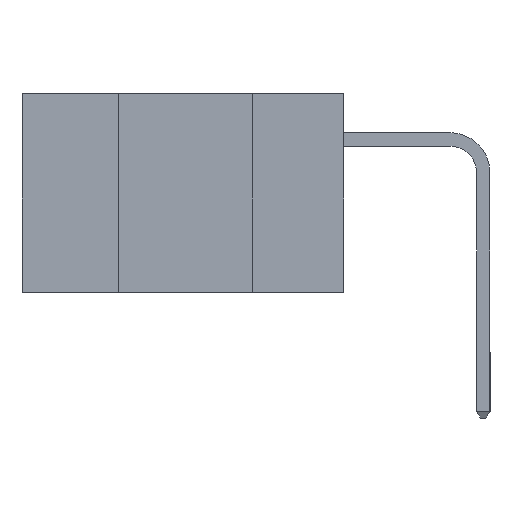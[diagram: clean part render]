
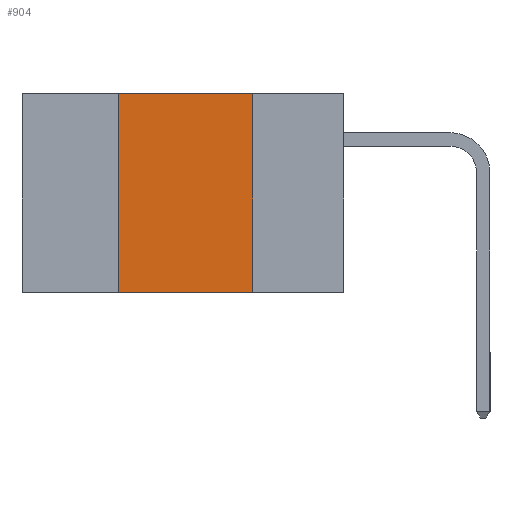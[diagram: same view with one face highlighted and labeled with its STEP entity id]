
A CAD part, left-side view. The second image highlights one B-rep face of the part: STEP entity #904.
In plain terms, the highlighted planar face has unit normal (-1, 0, 0).
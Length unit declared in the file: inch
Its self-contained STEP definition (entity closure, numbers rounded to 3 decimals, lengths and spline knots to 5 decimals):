
#88 = CARTESIAN_POINT ( 'NONE',  ( 0., 0.17, -0.37 ) ) ;
#831 = DIRECTION ( 'NONE',  ( 1., 0., 0. ) ) ;
#833 = LINE ( 'NONE', #2860, #20976 ) ;
#904 = ADVANCED_FACE ( 'NONE', ( #4616 ), #12294, .F. ) ;
#2860 = CARTESIAN_POINT ( 'NONE',  ( 0., 0.17, -0.37 ) ) ;
#3346 = ORIENTED_EDGE ( 'NONE', *, *, #13549, .F. ) ;
#3560 = VERTEX_POINT ( 'NONE', #88 ) ;
#3604 = VECTOR ( 'NONE', #18724, 39.37008 ) ;
#3720 = LINE ( 'NONE', #15054, #3604 ) ;
#3820 = EDGE_CURVE ( 'NONE', #12799, #21347, #6678, .T. ) ;
#4525 = DIRECTION ( 'NONE',  ( 0., -1., 0. ) ) ;
#4616 = FACE_OUTER_BOUND ( 'NONE', #24104, .T. ) ;
#5555 = ORIENTED_EDGE ( 'NONE', *, *, #3820, .F. ) ;
#6678 = LINE ( 'NONE', #16099, #10545 ) ;
#9415 = LINE ( 'NONE', #13351, #17639 ) ;
#9416 = VERTEX_POINT ( 'NONE', #10700 ) ;
#10498 = DIRECTION ( 'NONE',  ( 0., 0., -1. ) ) ;
#10545 = VECTOR ( 'NONE', #4525, 39.37008 ) ;
#10700 = CARTESIAN_POINT ( 'NONE',  ( 0., 0.42, -0.37 ) ) ;
#12294 = PLANE ( 'NONE',  #18757 ) ;
#12799 = VERTEX_POINT ( 'NONE', #22615 ) ;
#13351 = CARTESIAN_POINT ( 'NONE',  ( 0., 0.6, -0.37 ) ) ;
#13549 = EDGE_CURVE ( 'NONE', #21347, #3560, #833, .T. ) ;
#15054 = CARTESIAN_POINT ( 'NONE',  ( 0., 0.42, -0.37 ) ) ;
#15356 = DIRECTION ( 'NONE',  ( 0., -1., 0. ) ) ;
#16099 = CARTESIAN_POINT ( 'NONE',  ( 0., 0.6, 0. ) ) ;
#16182 = DIRECTION ( 'NONE',  ( 0., 0., -1. ) ) ;
#16784 = ORIENTED_EDGE ( 'NONE', *, *, #22926, .F. ) ;
#17639 = VECTOR ( 'NONE', #15356, 39.37008 ) ;
#18724 = DIRECTION ( 'NONE',  ( 0., 0., 1. ) ) ;
#18757 = AXIS2_PLACEMENT_3D ( 'NONE', #20028, #831, #16182 ) ;
#20028 = CARTESIAN_POINT ( 'NONE',  ( 0., 0.6, 0. ) ) ;
#20795 = EDGE_CURVE ( 'NONE', #9416, #3560, #9415, .T. ) ;
#20976 = VECTOR ( 'NONE', #10498, 39.37008 ) ;
#21347 = VERTEX_POINT ( 'NONE', #21979 ) ;
#21979 = CARTESIAN_POINT ( 'NONE',  ( 0., 0.17, 0. ) ) ;
#22615 = CARTESIAN_POINT ( 'NONE',  ( 0., 0.42, 0. ) ) ;
#22926 = EDGE_CURVE ( 'NONE', #9416, #12799, #3720, .T. ) ;
#24019 = ORIENTED_EDGE ( 'NONE', *, *, #20795, .T. ) ;
#24104 = EDGE_LOOP ( 'NONE', ( #3346, #5555, #16784, #24019 ) ) ;
